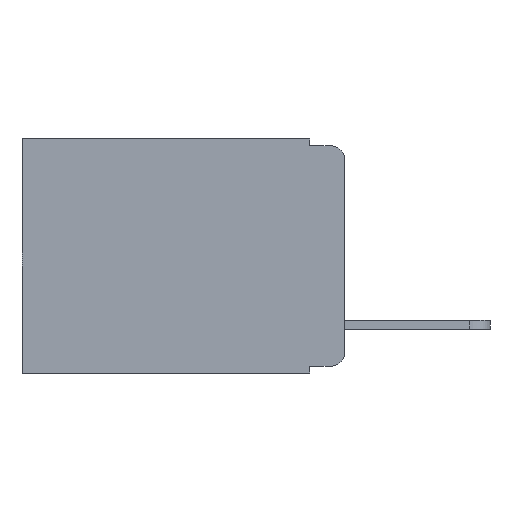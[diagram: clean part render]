
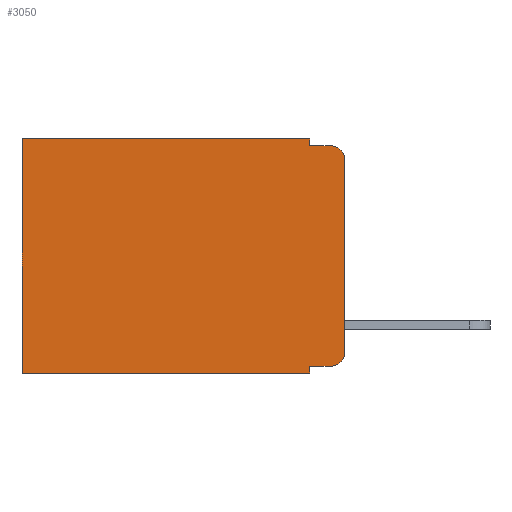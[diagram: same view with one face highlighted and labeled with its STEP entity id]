
A CAD part, left-side view. The second image highlights one B-rep face of the part: STEP entity #3050.
In plain terms, the highlighted planar face has unit normal (-1, 0, 0).
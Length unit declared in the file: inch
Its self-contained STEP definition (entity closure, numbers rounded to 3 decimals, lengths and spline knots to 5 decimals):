
#560 = CARTESIAN_POINT ( 'NONE',  ( 0.298, 0., 0. ) ) ;
#776 = LINE ( 'NONE', #7669, #7538 ) ;
#796 = EDGE_CURVE ( 'NONE', #10365, #7209, #9701, .T. ) ;
#895 = ORIENTED_EDGE ( 'NONE', *, *, #2070, .T. ) ;
#1251 = ORIENTED_EDGE ( 'NONE', *, *, #4837, .F. ) ;
#1450 = CARTESIAN_POINT ( 'NONE',  ( 0.298, 0.051, -0.01 ) ) ;
#1495 = VECTOR ( 'NONE', #4957, 39.37008 ) ;
#1526 = VERTEX_POINT ( 'NONE', #5808 ) ;
#1785 = EDGE_CURVE ( 'NONE', #4999, #3319, #8218, .T. ) ;
#1884 = VERTEX_POINT ( 'NONE', #7002 ) ;
#1915 = LINE ( 'NONE', #9010, #3725 ) ;
#2019 = LINE ( 'NONE', #9950, #1495 ) ;
#2029 = LINE ( 'NONE', #3049, #10660 ) ;
#2070 = EDGE_CURVE ( 'NONE', #9775, #1526, #7710, .T. ) ;
#2158 = ORIENTED_EDGE ( 'NONE', *, *, #796, .T. ) ;
#2176 = DIRECTION ( 'NONE',  ( 0., -1., 0. ) ) ;
#2387 = ORIENTED_EDGE ( 'NONE', *, *, #6665, .F. ) ;
#2690 = CIRCLE ( 'NONE', #10493, 0.02 ) ;
#2798 = CARTESIAN_POINT ( 'NONE',  ( 0.298, 0., -0.313 ) ) ;
#3045 = DIRECTION ( 'NONE',  ( 1., 0., 0. ) ) ;
#3049 = CARTESIAN_POINT ( 'NONE',  ( 0.298, 0., 0. ) ) ;
#3050 = ADVANCED_FACE ( 'NONE', ( #8191 ), #8058, .F. ) ;
#3161 = DIRECTION ( 'NONE',  ( 0., 0., -1. ) ) ;
#3298 = DIRECTION ( 'NONE',  ( 0., 0., -1. ) ) ;
#3319 = VERTEX_POINT ( 'NONE', #6751 ) ;
#3535 = DIRECTION ( 'NONE',  ( 0., 0., -1. ) ) ;
#3725 = VECTOR ( 'NONE', #3161, 39.37008 ) ;
#3803 = CARTESIAN_POINT ( 'NONE',  ( 0.298, 0.051, -0.333 ) ) ;
#3984 = AXIS2_PLACEMENT_3D ( 'NONE', #560, #3045, #10630 ) ;
#4098 = DIRECTION ( 'NONE',  ( -1., 0., 0. ) ) ;
#4418 = EDGE_CURVE ( 'NONE', #10365, #10071, #1915, .T. ) ;
#4783 = VERTEX_POINT ( 'NONE', #10513 ) ;
#4816 = VECTOR ( 'NONE', #8887, 39.37008 ) ;
#4837 = EDGE_CURVE ( 'NONE', #1884, #7209, #9625, .T. ) ;
#4865 = CARTESIAN_POINT ( 'NONE',  ( 0.298, 0.02, -0.313 ) ) ;
#4957 = DIRECTION ( 'NONE',  ( 0., 0., -1. ) ) ;
#4964 = AXIS2_PLACEMENT_3D ( 'NONE', #7718, #10256, #5224 ) ;
#4999 = VERTEX_POINT ( 'NONE', #8147 ) ;
#5077 = ORIENTED_EDGE ( 'NONE', *, *, #7101, .T. ) ;
#5142 = ORIENTED_EDGE ( 'NONE', *, *, #8719, .F. ) ;
#5224 = DIRECTION ( 'NONE',  ( 0., 0., -1. ) ) ;
#5624 = CARTESIAN_POINT ( 'NONE',  ( 0.298, 0.02, -0.01 ) ) ;
#5629 = EDGE_LOOP ( 'NONE', ( #9847, #2158, #1251, #2387, #9219, #6761, #5142, #9749, #895, #5077 ) ) ;
#5808 = CARTESIAN_POINT ( 'NONE',  ( 0.298, 0.02, -0.333 ) ) ;
#5864 = DIRECTION ( 'NONE',  ( 0., 0., -1. ) ) ;
#6665 = EDGE_CURVE ( 'NONE', #4783, #1884, #776, .T. ) ;
#6751 = CARTESIAN_POINT ( 'NONE',  ( 0.298, 0.473, -0.343 ) ) ;
#6761 = ORIENTED_EDGE ( 'NONE', *, *, #1785, .T. ) ;
#6971 = VERTEX_POINT ( 'NONE', #9711 ) ;
#6998 = VECTOR ( 'NONE', #2176, 39.37008 ) ;
#7002 = CARTESIAN_POINT ( 'NONE',  ( 0.298, 0.051, -0.01 ) ) ;
#7092 = LINE ( 'NONE', #7691, #8795 ) ;
#7101 = EDGE_CURVE ( 'NONE', #1526, #10071, #2690, .T. ) ;
#7209 = VERTEX_POINT ( 'NONE', #5624 ) ;
#7296 = CARTESIAN_POINT ( 'NONE',  ( 0.298, 0., -0.03 ) ) ;
#7349 = CARTESIAN_POINT ( 'NONE',  ( 0.298, 0.051, -0.333 ) ) ;
#7538 = VECTOR ( 'NONE', #5864, 39.37008 ) ;
#7578 = VECTOR ( 'NONE', #3535, 39.37008 ) ;
#7669 = CARTESIAN_POINT ( 'NONE',  ( 0.298, 0.051, 0. ) ) ;
#7691 = CARTESIAN_POINT ( 'NONE',  ( 0.298, 0., -0.343 ) ) ;
#7710 = LINE ( 'NONE', #3803, #4816 ) ;
#7718 = CARTESIAN_POINT ( 'NONE',  ( 0.298, 0.02, -0.03 ) ) ;
#7741 = EDGE_CURVE ( 'NONE', #4783, #4999, #2029, .T. ) ;
#7881 = EDGE_CURVE ( 'NONE', #9775, #6971, #2019, .T. ) ;
#8058 = PLANE ( 'NONE',  #3984 ) ;
#8121 = DIRECTION ( 'NONE',  ( 0., 1., 0. ) ) ;
#8147 = CARTESIAN_POINT ( 'NONE',  ( 0.298, 0.473, 0. ) ) ;
#8191 = FACE_OUTER_BOUND ( 'NONE', #5629, .T. ) ;
#8218 = LINE ( 'NONE', #8393, #7578 ) ;
#8393 = CARTESIAN_POINT ( 'NONE',  ( 0.298, 0.473, 0. ) ) ;
#8690 = DIRECTION ( 'NONE',  ( 0., 1., 0. ) ) ;
#8719 = EDGE_CURVE ( 'NONE', #6971, #3319, #7092, .T. ) ;
#8795 = VECTOR ( 'NONE', #8690, 39.37008 ) ;
#8887 = DIRECTION ( 'NONE',  ( 0., -1., 0. ) ) ;
#9010 = CARTESIAN_POINT ( 'NONE',  ( 0.298, 0., 0. ) ) ;
#9219 = ORIENTED_EDGE ( 'NONE', *, *, #7741, .T. ) ;
#9625 = LINE ( 'NONE', #1450, #6998 ) ;
#9701 = CIRCLE ( 'NONE', #4964, 0.02 ) ;
#9711 = CARTESIAN_POINT ( 'NONE',  ( 0.298, 0.051, -0.343 ) ) ;
#9749 = ORIENTED_EDGE ( 'NONE', *, *, #7881, .F. ) ;
#9775 = VERTEX_POINT ( 'NONE', #7349 ) ;
#9847 = ORIENTED_EDGE ( 'NONE', *, *, #4418, .F. ) ;
#9950 = CARTESIAN_POINT ( 'NONE',  ( 0.298, 0.051, 0. ) ) ;
#10071 = VERTEX_POINT ( 'NONE', #2798 ) ;
#10256 = DIRECTION ( 'NONE',  ( -1., 0., 0. ) ) ;
#10365 = VERTEX_POINT ( 'NONE', #7296 ) ;
#10493 = AXIS2_PLACEMENT_3D ( 'NONE', #4865, #4098, #3298 ) ;
#10513 = CARTESIAN_POINT ( 'NONE',  ( 0.298, 0.051, 0. ) ) ;
#10630 = DIRECTION ( 'NONE',  ( 0., 0., -1. ) ) ;
#10660 = VECTOR ( 'NONE', #8121, 39.37008 ) ;
